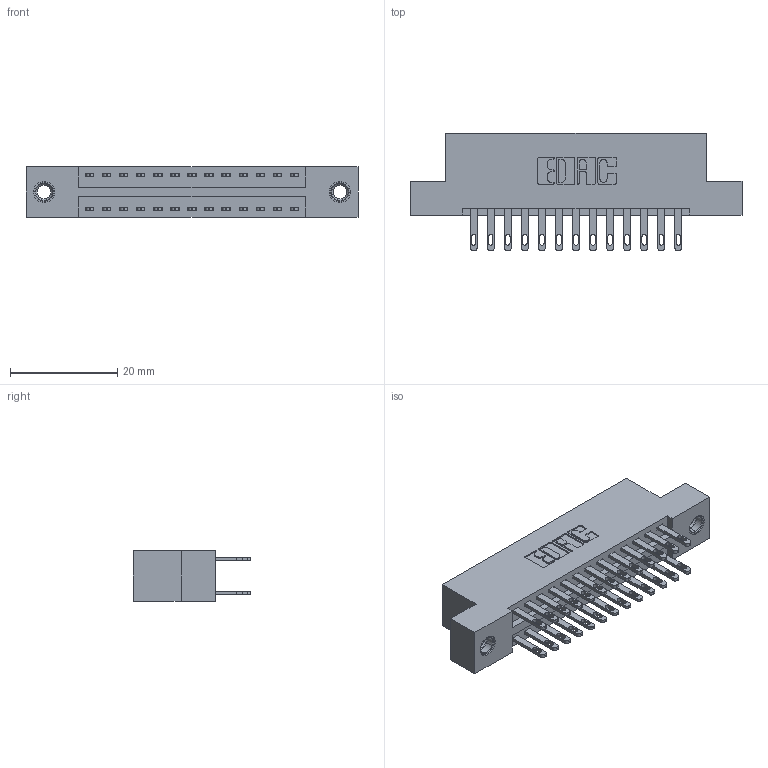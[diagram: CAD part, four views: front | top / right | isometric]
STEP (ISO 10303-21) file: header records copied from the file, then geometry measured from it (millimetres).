
FILE_DESCRIPTION (( 'STEP AP203' ), '1' );
FILE_NAME ('346-026-500-207.STEP', '2018-08-21T21:38:22', ( '' ), ( '' ), 'SwSTEP 2.0', 'SolidWorks 2016', '' );
FILE_SCHEMA (( 'CONFIG_CONTROL_DESIGN' ));
Length unit declared in the file: inch
Products named in the file (4): 346 Part_Flush Mounting Lugs - 0.156 Dia-TI; 345-292-001_345-293-100; 345-250-001_345-250-005-103; 346-026-500-207
Assembly tree (29 placements, depth 2):
  346-026-500-207
    346 Part_Flush Mounting Lugs - 0.156 Dia-TI
    345-292-001_345-293-100  x26
    345-250-001_345-250-005-103  x2
Bounding box: 61.85 x 21.84 x 9.4 mm (x, y, z)
Volume: 5871.7 mm3; surface area: 7921.2 mm2
Topology: 29 solids, 29 shells, 1430 faces, 4287 edges, 2850 vertices
Faces by surface type: plane 862, cylinder 552, cone 12, torus 4
Entity records: 13504 total; most frequent: CARTESIAN_POINT 2247, ORIENTED_EDGE 2174, DIRECTION 2061, EDGE_CURVE 1087, VECTOR 879, LINE 879, VERTEX_POINT 720, AXIS2_PLACEMENT_3D 591
